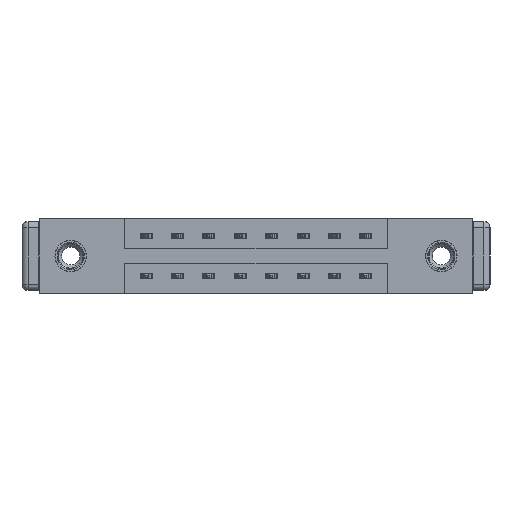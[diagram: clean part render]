
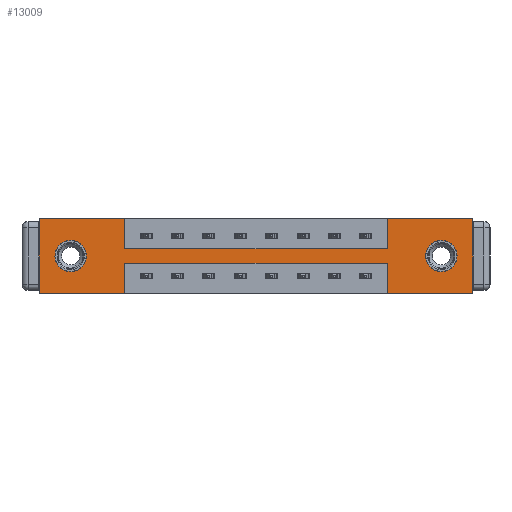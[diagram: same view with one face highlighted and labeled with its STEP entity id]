
A CAD part, front view. The second image highlights one B-rep face of the part: STEP entity #13009.
In plain terms, the highlighted planar face has unit normal (0, -1, 0).
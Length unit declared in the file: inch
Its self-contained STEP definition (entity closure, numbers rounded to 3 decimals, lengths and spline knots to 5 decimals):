
#71 = VERTEX_POINT ( 'NONE', #6259 ) ;
#77 = ORIENTED_EDGE ( 'NONE', *, *, #11484, .T. ) ;
#236 = EDGE_LOOP ( 'NONE', ( #1567, #10051, #1422, #13026, #10121, #3783, #1450, #6658, #5356, #1574, #4984, #5333 ) ) ;
#284 = LINE ( 'NONE', #11331, #3339 ) ;
#678 = VERTEX_POINT ( 'NONE', #12967 ) ;
#846 = LINE ( 'NONE', #8036, #12613 ) ;
#937 = VECTOR ( 'NONE', #3742, 39.37008 ) ;
#1250 = LINE ( 'NONE', #2646, #937 ) ;
#1312 = DIRECTION ( 'NONE',  ( 0., 1., 0. ) ) ;
#1422 = ORIENTED_EDGE ( 'NONE', *, *, #3294, .F. ) ;
#1450 = ORIENTED_EDGE ( 'NONE', *, *, #10289, .F. ) ;
#1492 = VERTEX_POINT ( 'NONE', #12168 ) ;
#1557 = EDGE_CURVE ( 'NONE', #11152, #11403, #5378, .T. ) ;
#1567 = ORIENTED_EDGE ( 'NONE', *, *, #2305, .F. ) ;
#1574 = ORIENTED_EDGE ( 'NONE', *, *, #3581, .F. ) ;
#1624 = CARTESIAN_POINT ( 'NONE',  ( 2.154, 0., -0.37 ) ) ;
#1642 = CARTESIAN_POINT ( 'NONE',  ( 0.425, 0., -0.22 ) ) ;
#1675 = CARTESIAN_POINT ( 'NONE',  ( 0., 0., 0. ) ) ;
#1722 = CARTESIAN_POINT ( 'NONE',  ( 1.729, 0., 0. ) ) ;
#1789 = CARTESIAN_POINT ( 'NONE',  ( 1.999, 0., -0.107 ) ) ;
#1914 = VERTEX_POINT ( 'NONE', #5840 ) ;
#2130 = VECTOR ( 'NONE', #6091, 39.37008 ) ;
#2166 = LINE ( 'NONE', #6102, #10725 ) ;
#2253 = VECTOR ( 'NONE', #9860, 39.37008 ) ;
#2282 = LINE ( 'NONE', #1675, #6971 ) ;
#2305 = EDGE_CURVE ( 'NONE', #3649, #2785, #2166, .T. ) ;
#2329 = AXIS2_PLACEMENT_3D ( 'NONE', #2528, #7589, #2396 ) ;
#2396 = DIRECTION ( 'NONE',  ( 0., 0., 1. ) ) ;
#2528 = CARTESIAN_POINT ( 'NONE',  ( 0.155, 0., -0.185 ) ) ;
#2555 = CARTESIAN_POINT ( 'NONE',  ( 1.729, 0., -0.22 ) ) ;
#2584 = VERTEX_POINT ( 'NONE', #8518 ) ;
#2646 = CARTESIAN_POINT ( 'NONE',  ( 0.425, 0., 0. ) ) ;
#2745 = VERTEX_POINT ( 'NONE', #2555 ) ;
#2785 = VERTEX_POINT ( 'NONE', #6779 ) ;
#2933 = DIRECTION ( 'NONE',  ( -1., 0., 0. ) ) ;
#3274 = LINE ( 'NONE', #8754, #8474 ) ;
#3294 = EDGE_CURVE ( 'NONE', #11662, #2745, #12953, .T. ) ;
#3339 = VECTOR ( 'NONE', #5980, 39.37008 ) ;
#3344 = LINE ( 'NONE', #1642, #2253 ) ;
#3370 = VECTOR ( 'NONE', #6740, 39.37008 ) ;
#3459 = EDGE_LOOP ( 'NONE', ( #77, #6355 ) ) ;
#3520 = VERTEX_POINT ( 'NONE', #1624 ) ;
#3581 = EDGE_CURVE ( 'NONE', #2584, #71, #2282, .T. ) ;
#3649 = VERTEX_POINT ( 'NONE', #4769 ) ;
#3742 = DIRECTION ( 'NONE',  ( 0., 0., -1. ) ) ;
#3757 = CARTESIAN_POINT ( 'NONE',  ( 1.729, 0., -0.37 ) ) ;
#3783 = ORIENTED_EDGE ( 'NONE', *, *, #6630, .F. ) ;
#3818 = CARTESIAN_POINT ( 'NONE',  ( 1.999, 0., -0.263 ) ) ;
#3879 = CIRCLE ( 'NONE', #10467, 0.078 ) ;
#3895 = DIRECTION ( 'NONE',  ( 0., 0., -1. ) ) ;
#3984 = CIRCLE ( 'NONE', #10424, 0.078 ) ;
#4033 = DIRECTION ( 'NONE',  ( 1., 0., 0. ) ) ;
#4248 = CARTESIAN_POINT ( 'NONE',  ( 0., 0., 0. ) ) ;
#4284 = VERTEX_POINT ( 'NONE', #6785 ) ;
#4456 = LINE ( 'NONE', #9683, #6723 ) ;
#4605 = FACE_BOUND ( 'NONE', #8809, .T. ) ;
#4692 = VECTOR ( 'NONE', #10445, 39.37008 ) ;
#4769 = CARTESIAN_POINT ( 'NONE',  ( 0.425, 0., -0.22 ) ) ;
#4827 = LINE ( 'NONE', #11093, #3370 ) ;
#4849 = LINE ( 'NONE', #10282, #2130 ) ;
#4969 = DIRECTION ( 'NONE',  ( 0., 1., 0. ) ) ;
#4984 = ORIENTED_EDGE ( 'NONE', *, *, #6011, .F. ) ;
#5237 = EDGE_CURVE ( 'NONE', #2785, #8932, #4849, .T. ) ;
#5291 = ORIENTED_EDGE ( 'NONE', *, *, #5317, .T. ) ;
#5317 = EDGE_CURVE ( 'NONE', #11403, #11152, #3879, .T. ) ;
#5333 = ORIENTED_EDGE ( 'NONE', *, *, #5237, .F. ) ;
#5356 = ORIENTED_EDGE ( 'NONE', *, *, #11944, .F. ) ;
#5378 = CIRCLE ( 'NONE', #8262, 0.078 ) ;
#5506 = EDGE_CURVE ( 'NONE', #3520, #11662, #846, .T. ) ;
#5830 = EDGE_CURVE ( 'NONE', #1492, #12271, #11487, .T. ) ;
#5840 = CARTESIAN_POINT ( 'NONE',  ( 2.154, 0., 0. ) ) ;
#5922 = CARTESIAN_POINT ( 'NONE',  ( 1.999, 0., -0.185 ) ) ;
#5980 = DIRECTION ( 'NONE',  ( 1., 0., 0. ) ) ;
#6011 = EDGE_CURVE ( 'NONE', #8932, #2584, #4827, .T. ) ;
#6071 = CARTESIAN_POINT ( 'NONE',  ( 0., 0., -0.37 ) ) ;
#6091 = DIRECTION ( 'NONE',  ( -1., 0., 0. ) ) ;
#6102 = CARTESIAN_POINT ( 'NONE',  ( 0.425, 0., -0.37 ) ) ;
#6186 = DIRECTION ( 'NONE',  ( 0., 0., -1. ) ) ;
#6233 = FACE_OUTER_BOUND ( 'NONE', #236, .T. ) ;
#6259 = CARTESIAN_POINT ( 'NONE',  ( 0.425, 0., 0. ) ) ;
#6264 = CARTESIAN_POINT ( 'NONE',  ( 1.729, 0., -0.37 ) ) ;
#6355 = ORIENTED_EDGE ( 'NONE', *, *, #5830, .T. ) ;
#6630 = EDGE_CURVE ( 'NONE', #12624, #1914, #11464, .T. ) ;
#6658 = ORIENTED_EDGE ( 'NONE', *, *, #11201, .F. ) ;
#6723 = VECTOR ( 'NONE', #10794, 39.37008 ) ;
#6740 = DIRECTION ( 'NONE',  ( 0., 0., 1. ) ) ;
#6779 = CARTESIAN_POINT ( 'NONE',  ( 0.425, 0., -0.37 ) ) ;
#6785 = CARTESIAN_POINT ( 'NONE',  ( 0.425, 0., -0.15 ) ) ;
#6889 = EDGE_CURVE ( 'NONE', #2745, #3649, #3344, .T. ) ;
#6971 = VECTOR ( 'NONE', #4033, 39.37008 ) ;
#7001 = PLANE ( 'NONE',  #7245 ) ;
#7215 = DIRECTION ( 'NONE',  ( 1., 0., 0. ) ) ;
#7245 = AXIS2_PLACEMENT_3D ( 'NONE', #6071, #13328, #6186 ) ;
#7506 = CARTESIAN_POINT ( 'NONE',  ( 0.155, 0., -0.185 ) ) ;
#7549 = DIRECTION ( 'NONE',  ( 0., 0., 1. ) ) ;
#7589 = DIRECTION ( 'NONE',  ( 0., 1., 0. ) ) ;
#7905 = ORIENTED_EDGE ( 'NONE', *, *, #1557, .T. ) ;
#8036 = CARTESIAN_POINT ( 'NONE',  ( 0., 0., -0.37 ) ) ;
#8262 = AXIS2_PLACEMENT_3D ( 'NONE', #5922, #4969, #3895 ) ;
#8406 = CARTESIAN_POINT ( 'NONE',  ( 0.155, 0., -0.107 ) ) ;
#8474 = VECTOR ( 'NONE', #11861, 39.37008 ) ;
#8518 = CARTESIAN_POINT ( 'NONE',  ( 0., 0., 0. ) ) ;
#8754 = CARTESIAN_POINT ( 'NONE',  ( 1.729, 0., 0. ) ) ;
#8809 = EDGE_LOOP ( 'NONE', ( #7905, #5291 ) ) ;
#8932 = VERTEX_POINT ( 'NONE', #12718 ) ;
#9683 = CARTESIAN_POINT ( 'NONE',  ( 2.154, 0., 0. ) ) ;
#9684 = DIRECTION ( 'NONE',  ( 0., 0., -1. ) ) ;
#9860 = DIRECTION ( 'NONE',  ( -1., 0., 0. ) ) ;
#10051 = ORIENTED_EDGE ( 'NONE', *, *, #6889, .F. ) ;
#10121 = ORIENTED_EDGE ( 'NONE', *, *, #12785, .F. ) ;
#10156 = DIRECTION ( 'NONE',  ( 0., 0., -1. ) ) ;
#10282 = CARTESIAN_POINT ( 'NONE',  ( 0., 0., -0.37 ) ) ;
#10289 = EDGE_CURVE ( 'NONE', #678, #12624, #3274, .T. ) ;
#10424 = AXIS2_PLACEMENT_3D ( 'NONE', #7506, #1312, #7549 ) ;
#10445 = DIRECTION ( 'NONE',  ( 0., 0., 1. ) ) ;
#10467 = AXIS2_PLACEMENT_3D ( 'NONE', #11657, #10661, #9684 ) ;
#10661 = DIRECTION ( 'NONE',  ( 0., 1., 0. ) ) ;
#10725 = VECTOR ( 'NONE', #10156, 39.37008 ) ;
#10794 = DIRECTION ( 'NONE',  ( 0., 0., -1. ) ) ;
#11084 = FACE_BOUND ( 'NONE', #3459, .T. ) ;
#11093 = CARTESIAN_POINT ( 'NONE',  ( 0., 0., 0. ) ) ;
#11152 = VERTEX_POINT ( 'NONE', #1789 ) ;
#11201 = EDGE_CURVE ( 'NONE', #4284, #678, #284, .T. ) ;
#11331 = CARTESIAN_POINT ( 'NONE',  ( 0.425, 0., -0.15 ) ) ;
#11403 = VERTEX_POINT ( 'NONE', #3818 ) ;
#11464 = LINE ( 'NONE', #4248, #11930 ) ;
#11484 = EDGE_CURVE ( 'NONE', #12271, #1492, #3984, .T. ) ;
#11487 = CIRCLE ( 'NONE', #2329, 0.078 ) ;
#11657 = CARTESIAN_POINT ( 'NONE',  ( 1.999, 0., -0.185 ) ) ;
#11662 = VERTEX_POINT ( 'NONE', #3757 ) ;
#11861 = DIRECTION ( 'NONE',  ( 0., 0., 1. ) ) ;
#11930 = VECTOR ( 'NONE', #7215, 39.37008 ) ;
#11944 = EDGE_CURVE ( 'NONE', #71, #4284, #1250, .T. ) ;
#12168 = CARTESIAN_POINT ( 'NONE',  ( 0.155, 0., -0.263 ) ) ;
#12271 = VERTEX_POINT ( 'NONE', #8406 ) ;
#12613 = VECTOR ( 'NONE', #2933, 39.37008 ) ;
#12624 = VERTEX_POINT ( 'NONE', #1722 ) ;
#12718 = CARTESIAN_POINT ( 'NONE',  ( 0., 0., -0.37 ) ) ;
#12785 = EDGE_CURVE ( 'NONE', #1914, #3520, #4456, .T. ) ;
#12953 = LINE ( 'NONE', #6264, #4692 ) ;
#12967 = CARTESIAN_POINT ( 'NONE',  ( 1.729, 0., -0.15 ) ) ;
#13009 = ADVANCED_FACE ( 'NONE', ( #4605, #11084, #6233 ), #7001, .T. ) ;
#13026 = ORIENTED_EDGE ( 'NONE', *, *, #5506, .F. ) ;
#13328 = DIRECTION ( 'NONE',  ( 0., -1., 0. ) ) ;
